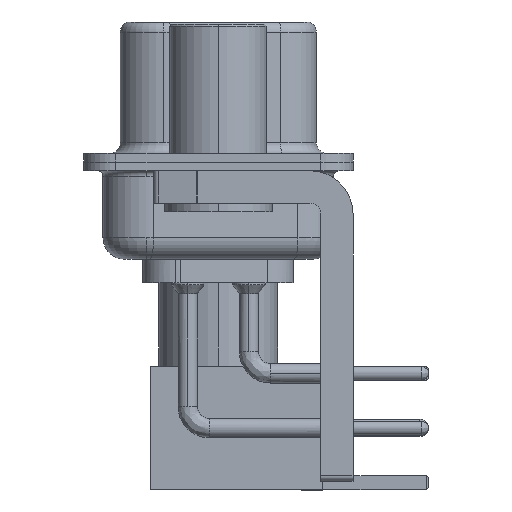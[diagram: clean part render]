
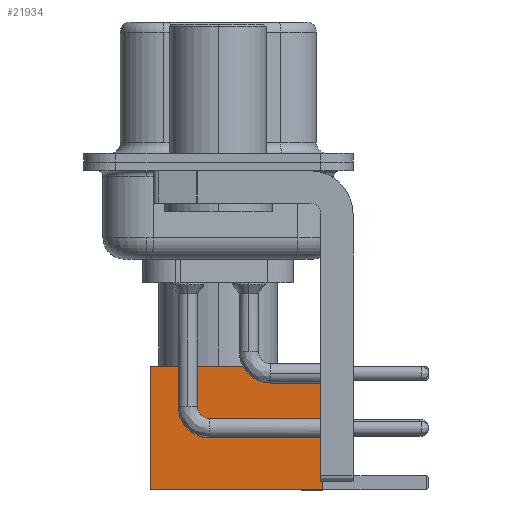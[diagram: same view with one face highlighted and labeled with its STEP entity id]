
A CAD part, left-side view. The second image highlights one B-rep face of the part: STEP entity #21934.
In plain terms, the highlighted face is planar.
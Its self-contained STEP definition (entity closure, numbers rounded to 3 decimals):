
#302 = LINE ( 'NONE', #2353, #13855 ) ;
#556 = EDGE_CURVE ( 'NONE', #27577, #12519, #24328, .T. ) ;
#2353 = CARTESIAN_POINT ( 'NONE',  ( 0., 2.875, 8. ) ) ;
#3641 = PLANE ( 'NONE',  #10076 ) ;
#3740 = ORIENTED_EDGE ( 'NONE', *, *, #556, .F. ) ;
#4269 = CARTESIAN_POINT ( 'NONE',  ( 2.875, 2.875, 0. ) ) ;
#4324 = CARTESIAN_POINT ( 'NONE',  ( -2.875, 2.875, 0. ) ) ;
#5068 = ORIENTED_EDGE ( 'NONE', *, *, #12575, .T. ) ;
#6123 = ORIENTED_EDGE ( 'NONE', *, *, #10164, .F. ) ;
#6503 = DIRECTION ( 'NONE',  ( -1., 0., 0. ) ) ;
#8319 = FACE_OUTER_BOUND ( 'NONE', #18284, .T. ) ;
#8512 = VERTEX_POINT ( 'NONE', #25840 ) ;
#10076 = AXIS2_PLACEMENT_3D ( 'NONE', #12251, #15000, #17199 ) ;
#10164 = EDGE_CURVE ( 'NONE', #8512, #27577, #302, .T. ) ;
#11120 = DIRECTION ( 'NONE',  ( 0., 0., -1. ) ) ;
#12251 = CARTESIAN_POINT ( 'NONE',  ( 2.875, 2.875, 0. ) ) ;
#12519 = VERTEX_POINT ( 'NONE', #28642 ) ;
#12575 = EDGE_CURVE ( 'NONE', #8512, #15522, #24277, .T. ) ;
#13201 = ORIENTED_EDGE ( 'NONE', *, *, #18448, .T. ) ;
#13713 = VECTOR ( 'NONE', #23787, 1000. ) ;
#13855 = VECTOR ( 'NONE', #18227, 1000. ) ;
#15000 = DIRECTION ( 'NONE',  ( 0., 1., 0. ) ) ;
#15522 = VERTEX_POINT ( 'NONE', #26191 ) ;
#15534 = LINE ( 'NONE', #26500, #25297 ) ;
#17199 = DIRECTION ( 'NONE',  ( 0., 0., 1. ) ) ;
#18227 = DIRECTION ( 'NONE',  ( -1., 0., 0. ) ) ;
#18284 = EDGE_LOOP ( 'NONE', ( #5068, #13201, #3740, #6123 ) ) ;
#18448 = EDGE_CURVE ( 'NONE', #15522, #12519, #15534, .T. ) ;
#21934 = ADVANCED_FACE ( 'NONE', ( #8319 ), #3641, .T. ) ;
#22301 = VECTOR ( 'NONE', #11120, 1000. ) ;
#23787 = DIRECTION ( 'NONE',  ( 0., 0., -1. ) ) ;
#24277 = LINE ( 'NONE', #4269, #22301 ) ;
#24328 = LINE ( 'NONE', #4324, #13713 ) ;
#25297 = VECTOR ( 'NONE', #6503, 1000. ) ;
#25840 = CARTESIAN_POINT ( 'NONE',  ( 2.875, 2.875, 8. ) ) ;
#26191 = CARTESIAN_POINT ( 'NONE',  ( 2.875, 2.875, 0. ) ) ;
#26500 = CARTESIAN_POINT ( 'NONE',  ( 0., 2.875, 0. ) ) ;
#27577 = VERTEX_POINT ( 'NONE', #28434 ) ;
#28434 = CARTESIAN_POINT ( 'NONE',  ( -2.875, 2.875, 8. ) ) ;
#28642 = CARTESIAN_POINT ( 'NONE',  ( -2.875, 2.875, 0. ) ) ;
